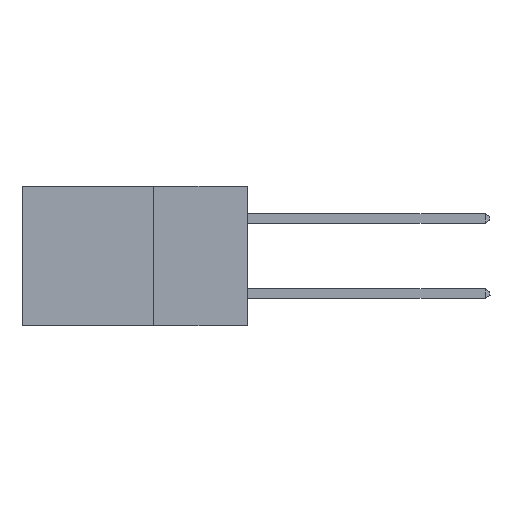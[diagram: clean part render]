
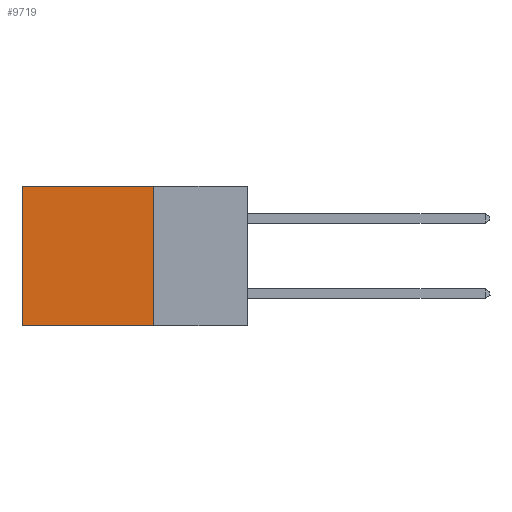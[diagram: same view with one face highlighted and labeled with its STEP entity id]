
A CAD part, left-side view. The second image highlights one B-rep face of the part: STEP entity #9719.
In plain terms, the highlighted planar face has unit normal (-1, 0, 0).
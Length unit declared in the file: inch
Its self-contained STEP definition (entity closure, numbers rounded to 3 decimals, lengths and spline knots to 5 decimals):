
#84 = EDGE_CURVE ( 'NONE', #353, #5372, #10720, .T. ) ;
#353 = VERTEX_POINT ( 'NONE', #6061 ) ;
#919 = ORIENTED_EDGE ( 'NONE', *, *, #9893, .F. ) ;
#948 = DIRECTION ( 'NONE',  ( 0., 1., 0. ) ) ;
#1233 = LINE ( 'NONE', #1663, #10947 ) ;
#1547 = CARTESIAN_POINT ( 'NONE',  ( 0.298, 0.25, -0.37 ) ) ;
#1655 = ORIENTED_EDGE ( 'NONE', *, *, #84, .F. ) ;
#1663 = CARTESIAN_POINT ( 'NONE',  ( 0.298, 0.25, 0. ) ) ;
#1853 = FACE_OUTER_BOUND ( 'NONE', #4171, .T. ) ;
#2130 = CARTESIAN_POINT ( 'NONE',  ( 0.298, 0.25, -0.37 ) ) ;
#2407 = DIRECTION ( 'NONE',  ( 0., 1., 0. ) ) ;
#3024 = DIRECTION ( 'NONE',  ( 1., 0., 0. ) ) ;
#4171 = EDGE_LOOP ( 'NONE', ( #8052, #919, #1655, #9688 ) ) ;
#4642 = VECTOR ( 'NONE', #6493, 39.37008 ) ;
#4990 = VERTEX_POINT ( 'NONE', #10341 ) ;
#5098 = AXIS2_PLACEMENT_3D ( 'NONE', #9818, #3024, #9772 ) ;
#5173 = VECTOR ( 'NONE', #2407, 39.37008 ) ;
#5372 = VERTEX_POINT ( 'NONE', #2130 ) ;
#5905 = VECTOR ( 'NONE', #9219, 39.37008 ) ;
#6061 = CARTESIAN_POINT ( 'NONE',  ( 0.298, 0.25, 0. ) ) ;
#6493 = DIRECTION ( 'NONE',  ( 0., 0., -1. ) ) ;
#7758 = LINE ( 'NONE', #1547, #5173 ) ;
#8052 = ORIENTED_EDGE ( 'NONE', *, *, #10888, .T. ) ;
#8493 = CARTESIAN_POINT ( 'NONE',  ( 0.298, 0.25, 0. ) ) ;
#8963 = VERTEX_POINT ( 'NONE', #11305 ) ;
#9219 = DIRECTION ( 'NONE',  ( 0., 0., -1. ) ) ;
#9669 = EDGE_CURVE ( 'NONE', #353, #8963, #1233, .T. ) ;
#9688 = ORIENTED_EDGE ( 'NONE', *, *, #9669, .T. ) ;
#9719 = ADVANCED_FACE ( 'NONE', ( #1853 ), #11635, .F. ) ;
#9772 = DIRECTION ( 'NONE',  ( 0., 0., -1. ) ) ;
#9818 = CARTESIAN_POINT ( 'NONE',  ( 0.298, 0.25, 0. ) ) ;
#9893 = EDGE_CURVE ( 'NONE', #5372, #4990, #7758, .T. ) ;
#10341 = CARTESIAN_POINT ( 'NONE',  ( 0.298, 0.6, -0.37 ) ) ;
#10445 = LINE ( 'NONE', #11287, #5905 ) ;
#10720 = LINE ( 'NONE', #8493, #4642 ) ;
#10888 = EDGE_CURVE ( 'NONE', #8963, #4990, #10445, .T. ) ;
#10947 = VECTOR ( 'NONE', #948, 39.37008 ) ;
#11287 = CARTESIAN_POINT ( 'NONE',  ( 0.298, 0.6, 0. ) ) ;
#11305 = CARTESIAN_POINT ( 'NONE',  ( 0.298, 0.6, 0. ) ) ;
#11635 = PLANE ( 'NONE',  #5098 ) ;
